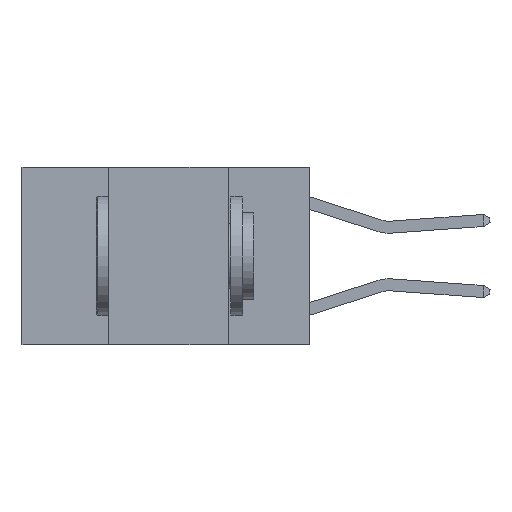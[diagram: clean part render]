
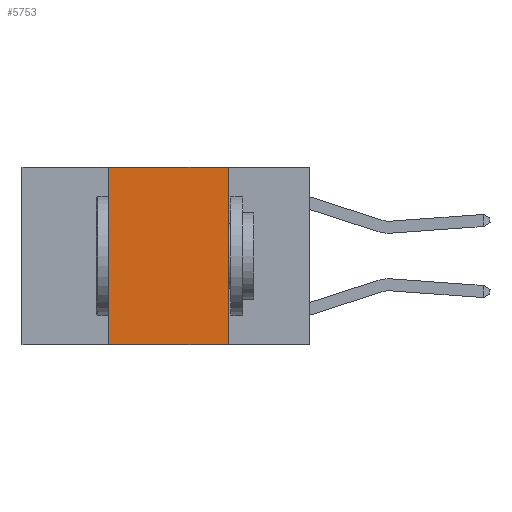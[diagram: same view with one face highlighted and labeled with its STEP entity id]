
A CAD part, left-side view. The second image highlights one B-rep face of the part: STEP entity #5753.
In plain terms, the highlighted planar face has unit normal (-1, 0, 0).
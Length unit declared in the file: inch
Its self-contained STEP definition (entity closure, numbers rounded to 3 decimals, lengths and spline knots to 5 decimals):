
#206 = DIRECTION ( 'NONE',  ( 0., -1., 0. ) ) ;
#254 = ORIENTED_EDGE ( 'NONE', *, *, #7334, .F. ) ;
#1233 = VECTOR ( 'NONE', #17514, 39.37008 ) ;
#2477 = EDGE_LOOP ( 'NONE', ( #11394, #254, #20583, #17071 ) ) ;
#2582 = CARTESIAN_POINT ( 'NONE',  ( 0., 0.17, -0.37 ) ) ;
#2639 = LINE ( 'NONE', #20905, #1233 ) ;
#3290 = VERTEX_POINT ( 'NONE', #6254 ) ;
#3773 = LINE ( 'NONE', #10415, #19213 ) ;
#4401 = VECTOR ( 'NONE', #17777, 39.37008 ) ;
#4477 = CARTESIAN_POINT ( 'NONE',  ( 0., 0.6, 0. ) ) ;
#4642 = EDGE_CURVE ( 'NONE', #5523, #9823, #3773, .T. ) ;
#5052 = AXIS2_PLACEMENT_3D ( 'NONE', #4477, #9793, #21404 ) ;
#5523 = VERTEX_POINT ( 'NONE', #15489 ) ;
#5753 = ADVANCED_FACE ( 'NONE', ( #6317 ), #12972, .F. ) ;
#6254 = CARTESIAN_POINT ( 'NONE',  ( 0., 0.17, 0. ) ) ;
#6317 = FACE_OUTER_BOUND ( 'NONE', #2477, .T. ) ;
#7046 = CARTESIAN_POINT ( 'NONE',  ( 0., 0.6, 0. ) ) ;
#7232 = CARTESIAN_POINT ( 'NONE',  ( 0., 0.42, 0. ) ) ;
#7334 = EDGE_CURVE ( 'NONE', #20854, #3290, #13608, .T. ) ;
#9793 = DIRECTION ( 'NONE',  ( 1., 0., 0. ) ) ;
#9823 = VERTEX_POINT ( 'NONE', #2582 ) ;
#10415 = CARTESIAN_POINT ( 'NONE',  ( 0., 0.6, -0.37 ) ) ;
#11063 = CARTESIAN_POINT ( 'NONE',  ( 0., 0.42, 0. ) ) ;
#11394 = ORIENTED_EDGE ( 'NONE', *, *, #19379, .F. ) ;
#12972 = PLANE ( 'NONE',  #5052 ) ;
#13608 = LINE ( 'NONE', #7046, #14591 ) ;
#14591 = VECTOR ( 'NONE', #206, 39.37008 ) ;
#15229 = DIRECTION ( 'NONE',  ( 0., -1., 0. ) ) ;
#15489 = CARTESIAN_POINT ( 'NONE',  ( 0., 0.42, -0.37 ) ) ;
#17071 = ORIENTED_EDGE ( 'NONE', *, *, #4642, .T. ) ;
#17514 = DIRECTION ( 'NONE',  ( 0., 0., -1. ) ) ;
#17777 = DIRECTION ( 'NONE',  ( 0., 0., 1. ) ) ;
#19213 = VECTOR ( 'NONE', #15229, 39.37008 ) ;
#19379 = EDGE_CURVE ( 'NONE', #3290, #9823, #2639, .T. ) ;
#19902 = LINE ( 'NONE', #11063, #4401 ) ;
#20583 = ORIENTED_EDGE ( 'NONE', *, *, #20930, .F. ) ;
#20854 = VERTEX_POINT ( 'NONE', #7232 ) ;
#20905 = CARTESIAN_POINT ( 'NONE',  ( 0., 0.17, 0. ) ) ;
#20930 = EDGE_CURVE ( 'NONE', #5523, #20854, #19902, .T. ) ;
#21404 = DIRECTION ( 'NONE',  ( 0., 0., -1. ) ) ;
